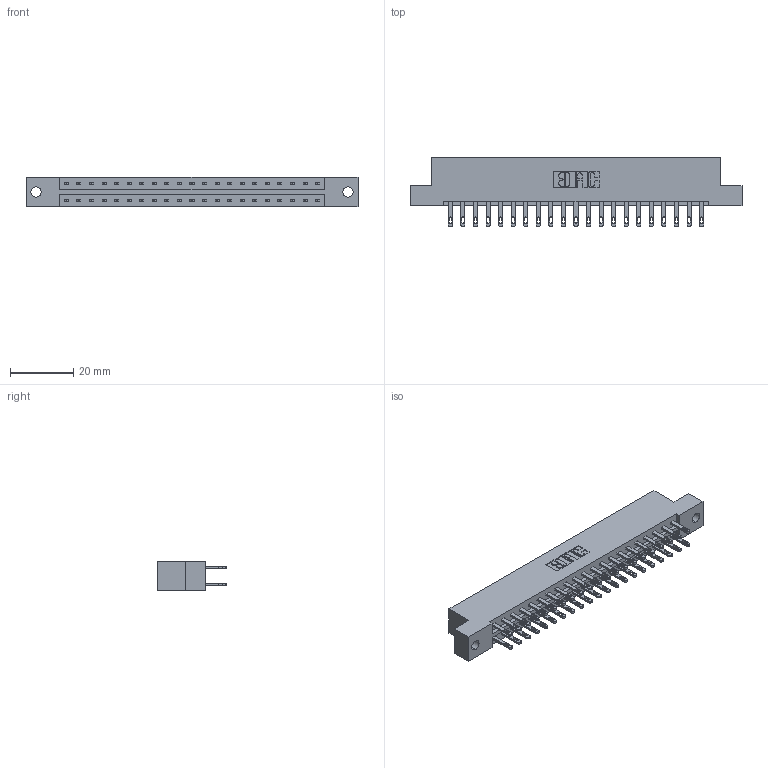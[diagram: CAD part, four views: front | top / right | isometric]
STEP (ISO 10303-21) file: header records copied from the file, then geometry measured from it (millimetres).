
FILE_DESCRIPTION (( 'STEP AP203' ), '1' );
FILE_NAME ('833-042-500-202.STEP', '2020-06-03T19:56:45', ( '' ), ( '' ), 'SwSTEP 2.0', 'SolidWorks 2020', '' );
FILE_SCHEMA (( 'CONFIG_CONTROL_DESIGN' ));
Length unit declared in the file: inch
Products named in the file (3): 833 Part_Flush - .128 Dia; 345-292-001_345-293-100; 833-042-500-202
Assembly tree (43 placements, depth 2):
  833-042-500-202
    833 Part_Flush - .128 Dia
    345-292-001_345-293-100  x42
Bounding box: 104.75 x 21.85 x 9.4 mm (x, y, z)
Volume: 10589.6 mm3; surface area: 12482.8 mm2
Topology: 43 solids, 43 shells, 2130 faces, 6485 edges, 4322 vertices
Faces by surface type: plane 1330, cylinder 800
Entity records: 16159 total; most frequent: CARTESIAN_POINT 2702, ORIENTED_EDGE 2638, DIRECTION 2347, EDGE_CURVE 1319, VECTOR 1187, LINE 1187, VERTEX_POINT 878, AXIS2_PLACEMENT_3D 580
